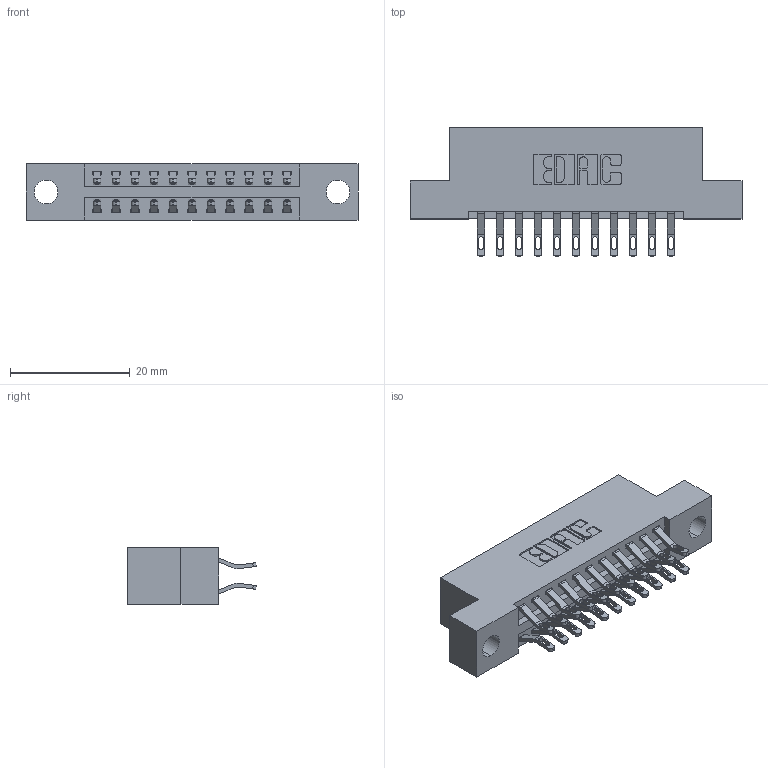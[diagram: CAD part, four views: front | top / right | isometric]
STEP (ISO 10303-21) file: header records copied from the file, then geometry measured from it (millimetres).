
FILE_DESCRIPTION (( 'STEP AP203' ), '1' );
FILE_NAME ('396-022-555-204.STEP', '2019-10-30T03:54:15', ( '' ), ( '' ), 'SwSTEP 2.0', 'SolidWorks 2016', '' );
FILE_SCHEMA (( 'CONFIG_CONTROL_DESIGN' ));
Length unit declared in the file: inch
Products named in the file (3): 396-022-555-204; 346 Part_Flush Mounting Lugs - 0.156 Dia-TH; 345-292-001_555 Tail
Assembly tree (23 placements, depth 2):
  396-022-555-204
    346 Part_Flush Mounting Lugs - 0.156 Dia-TH
    345-292-001_555 Tail  x22
Bounding box: 55.5 x 21.46 x 9.4 mm (x, y, z)
Volume: 5147 mm3; surface area: 6628.5 mm2
Topology: 23 solids, 23 shells, 1398 faces, 4355 edges, 2902 vertices
Faces by surface type: plane 802, cylinder 596
Entity records: 11681 total; most frequent: CARTESIAN_POINT 2002, ORIENTED_EDGE 1906, DIRECTION 1785, EDGE_CURVE 953, VECTOR 757, LINE 757, VERTEX_POINT 634, AXIS2_PLACEMENT_3D 514
